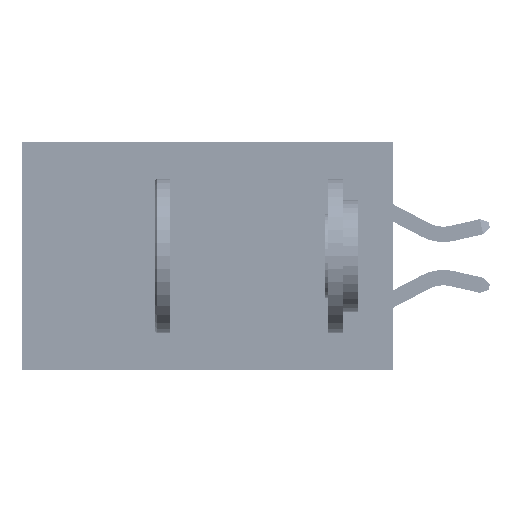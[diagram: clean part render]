
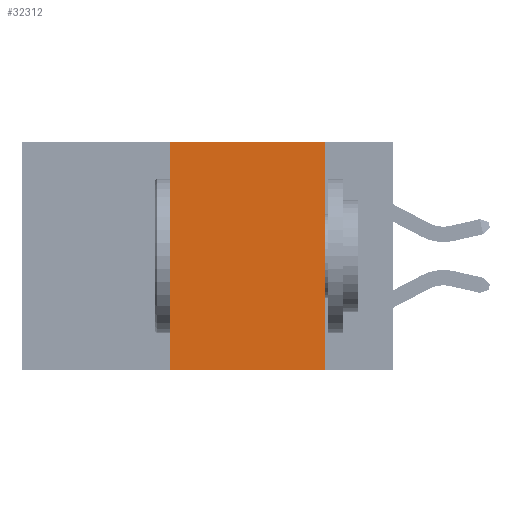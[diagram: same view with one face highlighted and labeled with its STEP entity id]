
A CAD part, left-side view. The second image highlights one B-rep face of the part: STEP entity #32312.
In plain terms, the highlighted planar face has unit normal (-1, 0, 0).
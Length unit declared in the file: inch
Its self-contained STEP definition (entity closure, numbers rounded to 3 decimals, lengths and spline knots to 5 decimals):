
#753 = CARTESIAN_POINT ( 'NONE',  ( 0., 0.36, 0. ) ) ;
#2974 = VERTEX_POINT ( 'NONE', #753 ) ;
#3322 = DIRECTION ( 'NONE',  ( 0., -1., 0. ) ) ;
#6311 = CARTESIAN_POINT ( 'NONE',  ( 0., 0.36, 0. ) ) ;
#9009 = DIRECTION ( 'NONE',  ( 0., 0., -1. ) ) ;
#10002 = DIRECTION ( 'NONE',  ( 0., 0., 1. ) ) ;
#10165 = ORIENTED_EDGE ( 'NONE', *, *, #46325, .F. ) ;
#13118 = EDGE_CURVE ( 'NONE', #16085, #36404, #36322, .T. ) ;
#13247 = PLANE ( 'NONE',  #37857 ) ;
#13957 = VECTOR ( 'NONE', #10002, 39.37008 ) ;
#15078 = CARTESIAN_POINT ( 'NONE',  ( 0., 0.36, -0.37 ) ) ;
#15344 = EDGE_CURVE ( 'NONE', #2974, #16085, #19970, .T. ) ;
#16085 = VERTEX_POINT ( 'NONE', #46937 ) ;
#16247 = CARTESIAN_POINT ( 'NONE',  ( 0., 0.11, -0.37 ) ) ;
#16484 = ORIENTED_EDGE ( 'NONE', *, *, #15344, .F. ) ;
#17869 = CARTESIAN_POINT ( 'NONE',  ( 0., 0.6, 0. ) ) ;
#19970 = LINE ( 'NONE', #17869, #36872 ) ;
#20603 = DIRECTION ( 'NONE',  ( 0., 0., -1. ) ) ;
#22791 = VERTEX_POINT ( 'NONE', #15078 ) ;
#23658 = LINE ( 'NONE', #6311, #13957 ) ;
#26785 = FACE_OUTER_BOUND ( 'NONE', #28246, .T. ) ;
#28246 = EDGE_LOOP ( 'NONE', ( #36253, #16484, #10165, #38534 ) ) ;
#29014 = DIRECTION ( 'NONE',  ( 0., -1., 0. ) ) ;
#32312 = ADVANCED_FACE ( 'NONE', ( #26785 ), #13247, .F. ) ;
#34431 = CARTESIAN_POINT ( 'NONE',  ( 0., 0.11, 0. ) ) ;
#36123 = CARTESIAN_POINT ( 'NONE',  ( 0., 0.6, -0.37 ) ) ;
#36253 = ORIENTED_EDGE ( 'NONE', *, *, #13118, .F. ) ;
#36322 = LINE ( 'NONE', #34431, #37440 ) ;
#36404 = VERTEX_POINT ( 'NONE', #16247 ) ;
#36750 = EDGE_CURVE ( 'NONE', #22791, #36404, #46616, .T. ) ;
#36872 = VECTOR ( 'NONE', #29014, 39.37008 ) ;
#37440 = VECTOR ( 'NONE', #9009, 39.37008 ) ;
#37857 = AXIS2_PLACEMENT_3D ( 'NONE', #38516, #42124, #20603 ) ;
#38235 = VECTOR ( 'NONE', #3322, 39.37008 ) ;
#38516 = CARTESIAN_POINT ( 'NONE',  ( 0., 0.6, 0. ) ) ;
#38534 = ORIENTED_EDGE ( 'NONE', *, *, #36750, .T. ) ;
#42124 = DIRECTION ( 'NONE',  ( 1., 0., 0. ) ) ;
#46325 = EDGE_CURVE ( 'NONE', #22791, #2974, #23658, .T. ) ;
#46616 = LINE ( 'NONE', #36123, #38235 ) ;
#46937 = CARTESIAN_POINT ( 'NONE',  ( 0., 0.11, 0. ) ) ;
